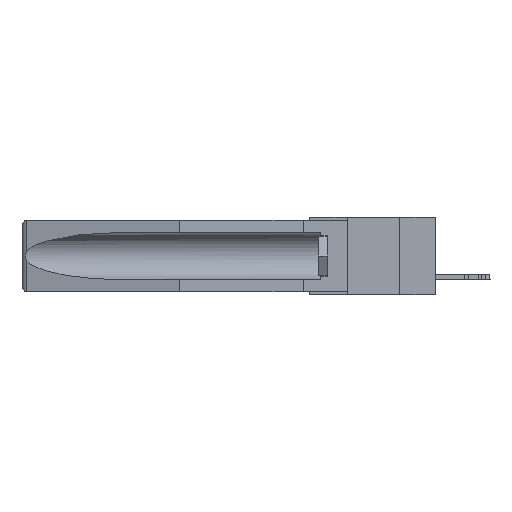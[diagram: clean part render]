
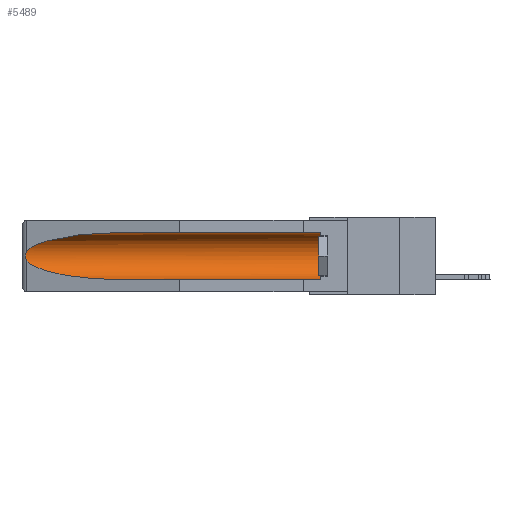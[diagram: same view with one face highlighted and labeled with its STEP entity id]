
A CAD part, left-side view. The second image highlights one B-rep face of the part: STEP entity #5489.
In plain terms, the highlighted cylindrical face has radius 2.857 mm (diameter 5.715 mm), a partial arc.
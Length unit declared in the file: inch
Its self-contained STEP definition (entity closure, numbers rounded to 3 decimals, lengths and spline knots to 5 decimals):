
#187 = CARTESIAN_POINT ( 'NONE',  ( 0.155, 0.126, -0.1715 ) ) ;
#206 = DIRECTION ( 'NONE',  ( 0., 0., 1. ) ) ;
#456 = CARTESIAN_POINT ( 'NONE',  ( 0.21114, 1.30732, -0.284 ) ) ;
#1162 = ORIENTED_EDGE ( 'NONE', *, *, #6786, .T. ) ;
#1579 = CARTESIAN_POINT ( 'NONE',  ( 0.26537, 1.52718, -0.19328 ) ) ;
#1829 = FACE_OUTER_BOUND ( 'NONE', #14635, .T. ) ;
#2338 = VERTEX_POINT ( 'NONE', #18253 ) ;
#2392 = CARTESIAN_POINT ( 'NONE',  ( 0.26654, 1.53092, -0.15636 ) ) ;
#3432 = EDGE_CURVE ( 'NONE', #10198, #15658, #28355, .T. ) ;
#4989 = ORIENTED_EDGE ( 'NONE', *, *, #3432, .T. ) ;
#5096 = ORIENTED_EDGE ( 'NONE', *, *, #5963, .F. ) ;
#5331 =( BOUNDED_CURVE ( )  B_SPLINE_CURVE ( 3, ( #5338, #15287, #456, #20002 ),
 .UNSPECIFIED., .F., .F. ) 
 B_SPLINE_CURVE_WITH_KNOTS ( ( 4, 4 ),
 ( 0.1948, 1.5708 ),
 .UNSPECIFIED. ) 
 CURVE ( )  GEOMETRIC_REPRESENTATION_ITEM ( )  RATIONAL_B_SPLINE_CURVE ( ( 1., 0.848, 0.848, 1. ) ) 
 REPRESENTATION_ITEM ( '' )  );
#5338 = CARTESIAN_POINT ( 'NONE',  ( 0.26537, 1.52718, -0.19328 ) ) ;
#5463 = CARTESIAN_POINT ( 'NONE',  ( 0.21114, 1.30732, -0.059 ) ) ;
#5489 = ADVANCED_FACE ( 'NONE', ( #1829 ), #27278, .F. ) ;
#5923 = DIRECTION ( 'NONE',  ( 0., 1., 0. ) ) ;
#5963 = EDGE_CURVE ( 'NONE', #28295, #30593, #17326, .T. ) ;
#6786 = EDGE_CURVE ( 'NONE', #15658, #30593, #5331, .T. ) ;
#7227 = CARTESIAN_POINT ( 'NONE',  ( 0.155, -0.30754, -0.1715 ) ) ;
#7492 = CARTESIAN_POINT ( 'NONE',  ( 0.2675, 1.53308, -0.17534 ) ) ;
#8090 = VECTOR ( 'NONE', #5923, 39.37008 ) ;
#10198 = VERTEX_POINT ( 'NONE', #26662 ) ;
#11680 = EDGE_CURVE ( 'NONE', #2338, #16607, #24283, .T. ) ;
#12356 = CARTESIAN_POINT ( 'NONE',  ( 0.26537, 1.52718, -0.14972 ) ) ;
#12570 = CARTESIAN_POINT ( 'NONE',  ( 0.26597, 1.52961, -0.15275 ) ) ;
#12600 = ORIENTED_EDGE ( 'NONE', *, *, #15849, .T. ) ;
#12821 = CARTESIAN_POINT ( 'NONE',  ( 0.155, 1.07973, -0.059 ) ) ;
#13814 = CARTESIAN_POINT ( 'NONE',  ( 0.155, -0.30754, -0.284 ) ) ;
#14635 = EDGE_LOOP ( 'NONE', ( #27884, #4989, #1162, #5096, #12600, #16644 ) ) ;
#14874 = CARTESIAN_POINT ( 'NONE',  ( 0.155, 1.07973, -0.284 ) ) ;
#15072 = CARTESIAN_POINT ( 'NONE',  ( 0.26537, 1.52718, -0.19328 ) ) ;
#15287 = CARTESIAN_POINT ( 'NONE',  ( 0.25451, 1.48313, -0.24835 ) ) ;
#15515 = CARTESIAN_POINT ( 'NONE',  ( 0.26537, 1.52718, -0.14972 ) ) ;
#15658 = VERTEX_POINT ( 'NONE', #1579 ) ;
#15662 = CARTESIAN_POINT ( 'NONE',  ( 0.155, -0.30754, -0.059 ) ) ;
#15849 = EDGE_CURVE ( 'NONE', #28295, #2338, #24229, .T. ) ;
#16607 = VERTEX_POINT ( 'NONE', #29427 ) ;
#16644 = ORIENTED_EDGE ( 'NONE', *, *, #11680, .T. ) ;
#16985 =( BOUNDED_CURVE ( )  B_SPLINE_CURVE ( 3, ( #12821, #5463, #30093, #15515 ),
 .UNSPECIFIED., .F., .F. ) 
 B_SPLINE_CURVE_WITH_KNOTS ( ( 4, 4 ),
 ( 4.71239, 6.08839 ),
 .UNSPECIFIED. ) 
 CURVE ( )  GEOMETRIC_REPRESENTATION_ITEM ( )  RATIONAL_B_SPLINE_CURVE ( ( 1., 0.848, 0.848, 1. ) ) 
 REPRESENTATION_ITEM ( '' )  );
#17326 = LINE ( 'NONE', #13814, #21170 ) ;
#17589 = DIRECTION ( 'NONE',  ( 0., -1., 0. ) ) ;
#18253 = CARTESIAN_POINT ( 'NONE',  ( 0.155, 0.126, -0.059 ) ) ;
#19782 = CARTESIAN_POINT ( 'NONE',  ( 0.2673, 1.5327, -0.16383 ) ) ;
#20002 = CARTESIAN_POINT ( 'NONE',  ( 0.155, 1.07973, -0.284 ) ) ;
#21170 = VECTOR ( 'NONE', #30981, 39.37008 ) ;
#22117 = DIRECTION ( 'NONE',  ( 0., 1., 0. ) ) ;
#23708 = AXIS2_PLACEMENT_3D ( 'NONE', #187, #17589, #29902 ) ;
#24229 = CIRCLE ( 'NONE', #23708, 0.1125 ) ;
#24283 = LINE ( 'NONE', #15662, #8090 ) ;
#24607 = CARTESIAN_POINT ( 'NONE',  ( 0.2675, 1.53308, -0.16763 ) ) ;
#25204 = CARTESIAN_POINT ( 'NONE',  ( 0.155, 0.126, -0.284 ) ) ;
#26662 = CARTESIAN_POINT ( 'NONE',  ( 0.26537, 1.52718, -0.14972 ) ) ;
#26793 = AXIS2_PLACEMENT_3D ( 'NONE', #7227, #22117, #206 ) ;
#27278 = CYLINDRICAL_SURFACE ( 'NONE', #26793, 0.1125 ) ;
#27884 = ORIENTED_EDGE ( 'NONE', *, *, #31806, .T. ) ;
#28295 = VERTEX_POINT ( 'NONE', #25204 ) ;
#28355 = B_SPLINE_CURVE_WITH_KNOTS ( 'NONE', 3,
 ( #12356, #12570, #2392, #19782, #24607, #7492, #31881, #29641, #29747, #15072 ),
 .UNSPECIFIED., .F., .F.,
 ( 4, 2, 2, 2, 4 ),
 ( 0., 0.00029, 0.00058, 0.00087, 0.00117 ),
 .UNSPECIFIED. ) ;
#29427 = CARTESIAN_POINT ( 'NONE',  ( 0.155, 1.07973, -0.059 ) ) ;
#29641 = CARTESIAN_POINT ( 'NONE',  ( 0.26655, 1.53094, -0.18657 ) ) ;
#29747 = CARTESIAN_POINT ( 'NONE',  ( 0.26597, 1.5296, -0.19026 ) ) ;
#29902 = DIRECTION ( 'NONE',  ( 0., 0., 1. ) ) ;
#30093 = CARTESIAN_POINT ( 'NONE',  ( 0.25451, 1.48313, -0.09465 ) ) ;
#30593 = VERTEX_POINT ( 'NONE', #14874 ) ;
#30981 = DIRECTION ( 'NONE',  ( 0., 1., 0. ) ) ;
#31806 = EDGE_CURVE ( 'NONE', #16607, #10198, #16985, .T. ) ;
#31881 = CARTESIAN_POINT ( 'NONE',  ( 0.2673, 1.53269, -0.17917 ) ) ;
